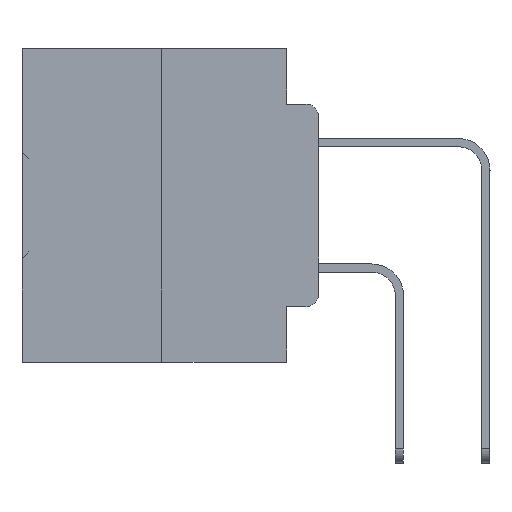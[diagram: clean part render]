
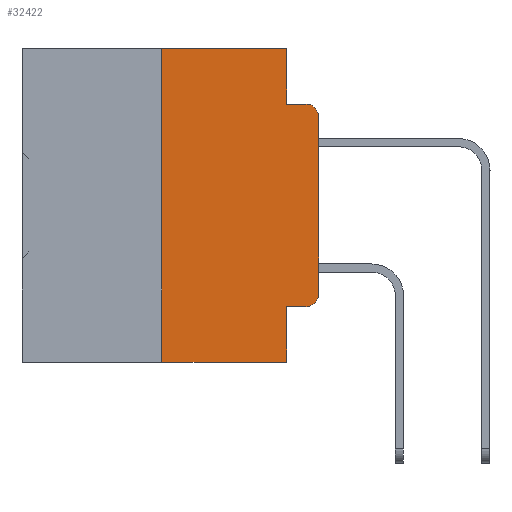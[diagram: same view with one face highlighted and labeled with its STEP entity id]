
A CAD part, left-side view. The second image highlights one B-rep face of the part: STEP entity #32422.
In plain terms, the highlighted planar face has unit normal (-1, 0, 0).
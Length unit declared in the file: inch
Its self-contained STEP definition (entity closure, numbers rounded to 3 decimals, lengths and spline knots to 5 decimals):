
#456 = CARTESIAN_POINT ( 'NONE',  ( 0., 0.051, 0. ) ) ;
#569 = ORIENTED_EDGE ( 'NONE', *, *, #26916, .T. ) ;
#2114 = LINE ( 'NONE', #20488, #30827 ) ;
#2226 = ORIENTED_EDGE ( 'NONE', *, *, #27725, .T. ) ;
#2903 = VECTOR ( 'NONE', #24763, 39.37008 ) ;
#3467 = VECTOR ( 'NONE', #8038, 39.37008 ) ;
#3600 = LINE ( 'NONE', #6691, #35380 ) ;
#4245 = CARTESIAN_POINT ( 'NONE',  ( 0., 0.02, -0.3915 ) ) ;
#4552 = EDGE_CURVE ( 'NONE', #5343, #28631, #39853, .T. ) ;
#4796 = DIRECTION ( 'NONE',  ( 0., -1., 0. ) ) ;
#5343 = VERTEX_POINT ( 'NONE', #22076 ) ;
#6144 = VERTEX_POINT ( 'NONE', #21677 ) ;
#6691 = CARTESIAN_POINT ( 'NONE',  ( 0., 0.473, 0. ) ) ;
#6898 = DIRECTION ( 'NONE',  ( 0., -1., 0. ) ) ;
#7265 = LINE ( 'NONE', #456, #11685 ) ;
#7341 = DIRECTION ( 'NONE',  ( -1., 0., 0. ) ) ;
#7840 = CIRCLE ( 'NONE', #33524, 0.02 ) ;
#8038 = DIRECTION ( 'NONE',  ( 0., 0., -1. ) ) ;
#8232 = EDGE_CURVE ( 'NONE', #6144, #9196, #27176, .T. ) ;
#8991 = AXIS2_PLACEMENT_3D ( 'NONE', #20629, #11334, #24130 ) ;
#9163 = DIRECTION ( 'NONE',  ( 1., 0., 0. ) ) ;
#9196 = VERTEX_POINT ( 'NONE', #34369 ) ;
#9927 = CARTESIAN_POINT ( 'NONE',  ( 0., 0., -0.1085 ) ) ;
#10440 = DIRECTION ( 'NONE',  ( 0., 0., -1. ) ) ;
#11140 = LINE ( 'NONE', #17727, #3467 ) ;
#11246 = CARTESIAN_POINT ( 'NONE',  ( 0., 0.051, -0.4115 ) ) ;
#11315 = VECTOR ( 'NONE', #34185, 39.37008 ) ;
#11334 = DIRECTION ( 'NONE',  ( -1., 0., 0. ) ) ;
#11469 = ORIENTED_EDGE ( 'NONE', *, *, #8232, .T. ) ;
#11685 = VECTOR ( 'NONE', #31831, 39.37008 ) ;
#12708 = EDGE_CURVE ( 'NONE', #27752, #19107, #34481, .T. ) ;
#13758 = CARTESIAN_POINT ( 'NONE',  ( 0., 0.051, 0. ) ) ;
#14765 = VERTEX_POINT ( 'NONE', #39367 ) ;
#15294 = AXIS2_PLACEMENT_3D ( 'NONE', #37437, #9163, #21759 ) ;
#15505 = ORIENTED_EDGE ( 'NONE', *, *, #20978, .F. ) ;
#15932 = ORIENTED_EDGE ( 'NONE', *, *, #4552, .T. ) ;
#17727 = CARTESIAN_POINT ( 'NONE',  ( 0., 0.051, 0. ) ) ;
#18444 = FACE_OUTER_BOUND ( 'NONE', #33264, .T. ) ;
#18985 = CARTESIAN_POINT ( 'NONE',  ( 0., 0.051, -0.4115 ) ) ;
#19107 = VERTEX_POINT ( 'NONE', #31822 ) ;
#20488 = CARTESIAN_POINT ( 'NONE',  ( 0., 0.051, -0.0885 ) ) ;
#20629 = CARTESIAN_POINT ( 'NONE',  ( 0., 0.02, -0.1085 ) ) ;
#20978 = EDGE_CURVE ( 'NONE', #25918, #35780, #7265, .T. ) ;
#21254 = CARTESIAN_POINT ( 'NONE',  ( 0., 0.02, -0.0885 ) ) ;
#21519 = CIRCLE ( 'NONE', #8991, 0.02 ) ;
#21590 = CARTESIAN_POINT ( 'NONE',  ( 0., 0.25, 0. ) ) ;
#21677 = CARTESIAN_POINT ( 'NONE',  ( 0., 0.25, -0.5 ) ) ;
#21759 = DIRECTION ( 'NONE',  ( 0., 0., -1. ) ) ;
#22076 = CARTESIAN_POINT ( 'NONE',  ( 0., 0., -0.3915 ) ) ;
#23542 = EDGE_CURVE ( 'NONE', #35780, #28919, #2114, .T. ) ;
#24130 = DIRECTION ( 'NONE',  ( 0., 0., -1. ) ) ;
#24468 = ORIENTED_EDGE ( 'NONE', *, *, #33790, .F. ) ;
#24763 = DIRECTION ( 'NONE',  ( 0., 0., 1. ) ) ;
#24847 = PLANE ( 'NONE',  #15294 ) ;
#25918 = VERTEX_POINT ( 'NONE', #13758 ) ;
#26398 = VECTOR ( 'NONE', #32966, 39.37008 ) ;
#26916 = EDGE_CURVE ( 'NONE', #28631, #28919, #21519, .T. ) ;
#27176 = LINE ( 'NONE', #36049, #26398 ) ;
#27725 = EDGE_CURVE ( 'NONE', #19107, #5343, #7840, .T. ) ;
#27752 = VERTEX_POINT ( 'NONE', #11246 ) ;
#28631 = VERTEX_POINT ( 'NONE', #9927 ) ;
#28919 = VERTEX_POINT ( 'NONE', #21254 ) ;
#30062 = EDGE_CURVE ( 'NONE', #27752, #9196, #11140, .T. ) ;
#30751 = CARTESIAN_POINT ( 'NONE',  ( 0., 0., 0. ) ) ;
#30827 = VECTOR ( 'NONE', #4796, 39.37008 ) ;
#31822 = CARTESIAN_POINT ( 'NONE',  ( 0., 0.02, -0.4115 ) ) ;
#31831 = DIRECTION ( 'NONE',  ( 0., 0., -1. ) ) ;
#31834 = ORIENTED_EDGE ( 'NONE', *, *, #23542, .F. ) ;
#32422 = ADVANCED_FACE ( 'NONE', ( #18444 ), #24847, .F. ) ;
#32966 = DIRECTION ( 'NONE',  ( 0., -1., 0. ) ) ;
#33264 = EDGE_LOOP ( 'NONE', ( #15932, #569, #31834, #15505, #24468, #36369, #11469, #34188, #34473, #2226 ) ) ;
#33524 = AXIS2_PLACEMENT_3D ( 'NONE', #4245, #7341, #10440 ) ;
#33790 = EDGE_CURVE ( 'NONE', #14765, #25918, #3600, .T. ) ;
#33975 = LINE ( 'NONE', #21590, #11315 ) ;
#34185 = DIRECTION ( 'NONE',  ( 0., 0., 1. ) ) ;
#34188 = ORIENTED_EDGE ( 'NONE', *, *, #30062, .F. ) ;
#34274 = CARTESIAN_POINT ( 'NONE',  ( 0., 0.051, -0.0885 ) ) ;
#34369 = CARTESIAN_POINT ( 'NONE',  ( 0., 0.051, -0.5 ) ) ;
#34473 = ORIENTED_EDGE ( 'NONE', *, *, #12708, .T. ) ;
#34481 = LINE ( 'NONE', #18985, #35775 ) ;
#35380 = VECTOR ( 'NONE', #6898, 39.37008 ) ;
#35775 = VECTOR ( 'NONE', #37980, 39.37008 ) ;
#35780 = VERTEX_POINT ( 'NONE', #34274 ) ;
#36049 = CARTESIAN_POINT ( 'NONE',  ( 0., 0.473, -0.5 ) ) ;
#36369 = ORIENTED_EDGE ( 'NONE', *, *, #39530, .F. ) ;
#37437 = CARTESIAN_POINT ( 'NONE',  ( 0., 0.473, 0. ) ) ;
#37980 = DIRECTION ( 'NONE',  ( 0., -1., 0. ) ) ;
#39367 = CARTESIAN_POINT ( 'NONE',  ( 0., 0.25, 0. ) ) ;
#39530 = EDGE_CURVE ( 'NONE', #6144, #14765, #33975, .T. ) ;
#39853 = LINE ( 'NONE', #30751, #2903 ) ;
